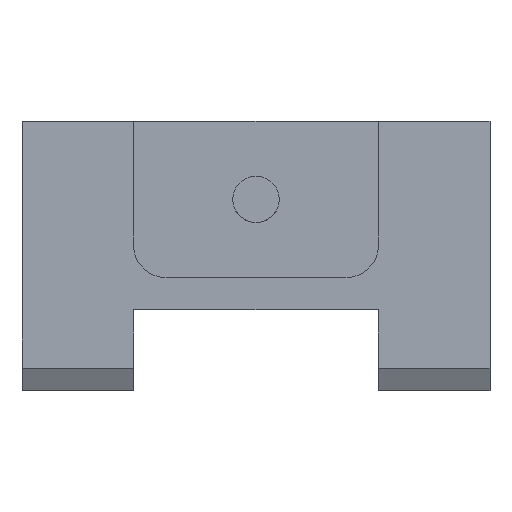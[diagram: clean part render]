
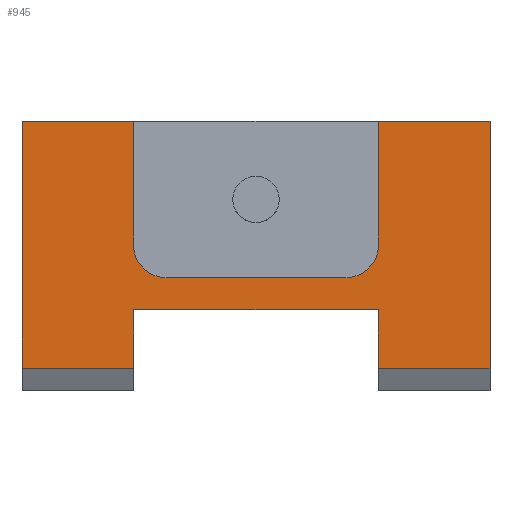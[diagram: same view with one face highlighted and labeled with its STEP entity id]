
A CAD part, front view. The second image highlights one B-rep face of the part: STEP entity #945.
In plain terms, the highlighted planar face has unit normal (0, -1, 0).
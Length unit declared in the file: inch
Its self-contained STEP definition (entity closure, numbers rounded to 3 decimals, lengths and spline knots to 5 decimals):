
#31 = LINE ( 'NONE', #756, #390 ) ;
#41 = EDGE_CURVE ( 'NONE', #1036, #1460, #516, .T. ) ;
#51 = VECTOR ( 'NONE', #1826, 39.37008 ) ;
#57 = LINE ( 'NONE', #1386, #876 ) ;
#76 = VERTEX_POINT ( 'NONE', #584 ) ;
#96 = CARTESIAN_POINT ( 'NONE',  ( -0.449, 0., -0.47359 ) ) ;
#110 = VECTOR ( 'NONE', #715, 39.37008 ) ;
#113 = ORIENTED_EDGE ( 'NONE', *, *, #724, .F. ) ;
#126 = DIRECTION ( 'NONE',  ( 0., -1., 0. ) ) ;
#137 = DIRECTION ( 'NONE',  ( 0., 0., -1. ) ) ;
#142 = DIRECTION ( 'NONE',  ( 1., 0., 0. ) ) ;
#170 = AXIS2_PLACEMENT_3D ( 'NONE', #1160, #1465, #550 ) ;
#218 = EDGE_CURVE ( 'NONE', #1460, #705, #1453, .T. ) ;
#229 = CARTESIAN_POINT ( 'NONE',  ( -0.235, 0., -0.2375 ) ) ;
#232 = VECTOR ( 'NONE', #1902, 39.37008 ) ;
#237 = ORIENTED_EDGE ( 'NONE', *, *, #247, .F. ) ;
#247 = EDGE_CURVE ( 'NONE', #898, #705, #897, .T. ) ;
#271 = EDGE_CURVE ( 'NONE', #932, #1186, #856, .T. ) ;
#278 = EDGE_CURVE ( 'NONE', #76, #898, #31, .T. ) ;
#279 = CARTESIAN_POINT ( 'NONE',  ( 0.1725, 0., -0.2375 ) ) ;
#281 = VERTEX_POINT ( 'NONE', #291 ) ;
#291 = CARTESIAN_POINT ( 'NONE',  ( -0.235, 0., 0. ) ) ;
#296 = ORIENTED_EDGE ( 'NONE', *, *, #374, .F. ) ;
#343 = EDGE_CURVE ( 'NONE', #1895, #76, #1516, .T. ) ;
#374 = EDGE_CURVE ( 'NONE', #281, #1895, #808, .T. ) ;
#390 = VECTOR ( 'NONE', #142, 39.37008 ) ;
#427 = DIRECTION ( 'NONE',  ( 0., 0., -1. ) ) ;
#433 = VECTOR ( 'NONE', #1569, 39.37008 ) ;
#462 = DIRECTION ( 'NONE',  ( -1., 0., 0. ) ) ;
#472 = EDGE_CURVE ( 'NONE', #281, #1913, #57, .T. ) ;
#474 = CARTESIAN_POINT ( 'NONE',  ( 0.235, 0., -0.2375 ) ) ;
#490 = ORIENTED_EDGE ( 'NONE', *, *, #472, .T. ) ;
#516 = LINE ( 'NONE', #1313, #110 ) ;
#529 = CARTESIAN_POINT ( 'NONE',  ( -0.449, 0., 0. ) ) ;
#548 = ORIENTED_EDGE ( 'NONE', *, *, #557, .T. ) ;
#550 = DIRECTION ( 'NONE',  ( 0., 0., 1. ) ) ;
#557 = EDGE_CURVE ( 'NONE', #1913, #958, #615, .T. ) ;
#573 = ORIENTED_EDGE ( 'NONE', *, *, #1500, .F. ) ;
#584 = CARTESIAN_POINT ( 'NONE',  ( -0.1725, 0., -0.3 ) ) ;
#596 = CARTESIAN_POINT ( 'NONE',  ( -0.235, 0., -0.362 ) ) ;
#615 = LINE ( 'NONE', #1550, #1382 ) ;
#641 = CARTESIAN_POINT ( 'NONE',  ( 0.449, 0., -0.47359 ) ) ;
#660 = CARTESIAN_POINT ( 'NONE',  ( -0.235, 0., -0.517 ) ) ;
#664 = VECTOR ( 'NONE', #137, 39.37008 ) ;
#673 = CARTESIAN_POINT ( 'NONE',  ( 0.235, 0., -0.47359 ) ) ;
#705 = VERTEX_POINT ( 'NONE', #474 ) ;
#715 = DIRECTION ( 'NONE',  ( -1., 0., 0. ) ) ;
#724 = EDGE_CURVE ( 'NONE', #1314, #958, #1352, .T. ) ;
#734 = ORIENTED_EDGE ( 'NONE', *, *, #775, .T. ) ;
#756 = CARTESIAN_POINT ( 'NONE',  ( 0., 0., -0.3 ) ) ;
#767 = CARTESIAN_POINT ( 'NONE',  ( 0.235, 0., 0. ) ) ;
#775 = EDGE_CURVE ( 'NONE', #1314, #932, #863, .T. ) ;
#796 = DIRECTION ( 'NONE',  ( -1., 0., 0. ) ) ;
#798 = DIRECTION ( 'NONE',  ( 0., 0., -1. ) ) ;
#808 = LINE ( 'NONE', #1502, #664 ) ;
#845 = DIRECTION ( 'NONE',  ( 0., 0., 1. ) ) ;
#856 = LINE ( 'NONE', #596, #1201 ) ;
#863 = LINE ( 'NONE', #660, #433 ) ;
#876 = VECTOR ( 'NONE', #462, 39.37008 ) ;
#884 = CARTESIAN_POINT ( 'NONE',  ( 0.235, 0., 0. ) ) ;
#886 = CARTESIAN_POINT ( 'NONE',  ( 0.449, 0., 0. ) ) ;
#891 = EDGE_CURVE ( 'NONE', #1810, #1186, #1432, .T. ) ;
#896 = VECTOR ( 'NONE', #796, 39.37008 ) ;
#897 = CIRCLE ( 'NONE', #1766, 0.0625 ) ;
#898 = VERTEX_POINT ( 'NONE', #1737 ) ;
#932 = VERTEX_POINT ( 'NONE', #1606 ) ;
#939 = AXIS2_PLACEMENT_3D ( 'NONE', #1048, #126, #1196 ) ;
#945 = ADVANCED_FACE ( 'NONE', ( #1801 ), #1006, .F. ) ;
#958 = VERTEX_POINT ( 'NONE', #96 ) ;
#1006 = PLANE ( 'NONE',  #170 ) ;
#1023 = VECTOR ( 'NONE', #845, 39.37008 ) ;
#1036 = VERTEX_POINT ( 'NONE', #886 ) ;
#1048 = CARTESIAN_POINT ( 'NONE',  ( -0.1725, 0., -0.2375 ) ) ;
#1054 = ORIENTED_EDGE ( 'NONE', *, *, #891, .F. ) ;
#1070 = VERTEX_POINT ( 'NONE', #1342 ) ;
#1160 = CARTESIAN_POINT ( 'NONE',  ( 0.449, 0., 0. ) ) ;
#1186 = VERTEX_POINT ( 'NONE', #1371 ) ;
#1196 = DIRECTION ( 'NONE',  ( 0., 0., -1. ) ) ;
#1201 = VECTOR ( 'NONE', #1359, 39.37008 ) ;
#1217 = LINE ( 'NONE', #1540, #51 ) ;
#1290 = CARTESIAN_POINT ( 'NONE',  ( 0.235, 0., -0.517 ) ) ;
#1297 = EDGE_CURVE ( 'NONE', #1070, #1810, #1344, .T. ) ;
#1308 = ORIENTED_EDGE ( 'NONE', *, *, #343, .F. ) ;
#1313 = CARTESIAN_POINT ( 'NONE',  ( 0.449, 0., 0. ) ) ;
#1314 = VERTEX_POINT ( 'NONE', #1698 ) ;
#1342 = CARTESIAN_POINT ( 'NONE',  ( 0.449, 0., -0.47359 ) ) ;
#1344 = LINE ( 'NONE', #641, #896 ) ;
#1350 = DIRECTION ( 'NONE',  ( 0., -1., 0. ) ) ;
#1352 = LINE ( 'NONE', #1703, #1742 ) ;
#1359 = DIRECTION ( 'NONE',  ( 1., 0., 0. ) ) ;
#1371 = CARTESIAN_POINT ( 'NONE',  ( 0.235, 0., -0.362 ) ) ;
#1382 = VECTOR ( 'NONE', #798, 39.37008 ) ;
#1386 = CARTESIAN_POINT ( 'NONE',  ( 0.449, 0., 0. ) ) ;
#1409 = DIRECTION ( 'NONE',  ( -1., 0., 0. ) ) ;
#1432 = LINE ( 'NONE', #1290, #1023 ) ;
#1453 = LINE ( 'NONE', #884, #232 ) ;
#1460 = VERTEX_POINT ( 'NONE', #767 ) ;
#1465 = DIRECTION ( 'NONE',  ( 0., 1., 0. ) ) ;
#1472 = ORIENTED_EDGE ( 'NONE', *, *, #1297, .F. ) ;
#1497 = ORIENTED_EDGE ( 'NONE', *, *, #278, .F. ) ;
#1500 = EDGE_CURVE ( 'NONE', #1036, #1070, #1217, .T. ) ;
#1502 = CARTESIAN_POINT ( 'NONE',  ( -0.235, 0., 0. ) ) ;
#1516 = CIRCLE ( 'NONE', #939, 0.0625 ) ;
#1540 = CARTESIAN_POINT ( 'NONE',  ( 0.449, 0., 0. ) ) ;
#1550 = CARTESIAN_POINT ( 'NONE',  ( -0.449, 0., 0. ) ) ;
#1569 = DIRECTION ( 'NONE',  ( 0., 0., 1. ) ) ;
#1606 = CARTESIAN_POINT ( 'NONE',  ( -0.235, 0., -0.362 ) ) ;
#1652 = EDGE_LOOP ( 'NONE', ( #734, #1908, #1054, #1472, #573, #1827, #1929, #237, #1497, #1308, #296, #490, #548, #113 ) ) ;
#1698 = CARTESIAN_POINT ( 'NONE',  ( -0.235, 0., -0.47359 ) ) ;
#1703 = CARTESIAN_POINT ( 'NONE',  ( 0.449, 0., -0.47359 ) ) ;
#1737 = CARTESIAN_POINT ( 'NONE',  ( 0.1725, 0., -0.3 ) ) ;
#1742 = VECTOR ( 'NONE', #1409, 39.37008 ) ;
#1766 = AXIS2_PLACEMENT_3D ( 'NONE', #279, #1350, #427 ) ;
#1801 = FACE_OUTER_BOUND ( 'NONE', #1652, .T. ) ;
#1810 = VERTEX_POINT ( 'NONE', #673 ) ;
#1826 = DIRECTION ( 'NONE',  ( 0., 0., -1. ) ) ;
#1827 = ORIENTED_EDGE ( 'NONE', *, *, #41, .T. ) ;
#1895 = VERTEX_POINT ( 'NONE', #229 ) ;
#1902 = DIRECTION ( 'NONE',  ( 0., 0., -1. ) ) ;
#1908 = ORIENTED_EDGE ( 'NONE', *, *, #271, .T. ) ;
#1913 = VERTEX_POINT ( 'NONE', #529 ) ;
#1929 = ORIENTED_EDGE ( 'NONE', *, *, #218, .T. ) ;
